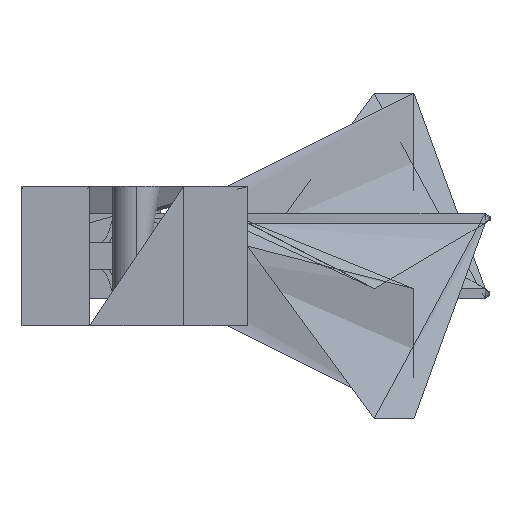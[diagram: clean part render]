
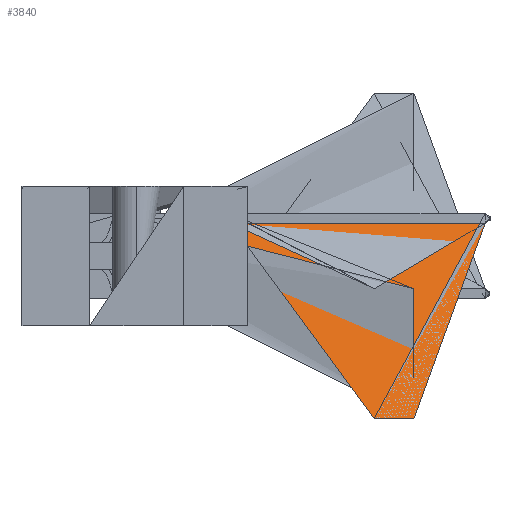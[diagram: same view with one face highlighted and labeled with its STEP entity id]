
A CAD part, left-side view. The second image highlights one B-rep face of the part: STEP entity #3840.
In plain terms, the highlighted face is planar.
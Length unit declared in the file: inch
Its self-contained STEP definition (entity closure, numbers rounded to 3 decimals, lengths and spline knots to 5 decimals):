
#121 = EDGE_CURVE ( 'NONE', #7818, #8210, #23582, .T. ) ;
#2265 = DIRECTION ( 'NONE',  ( -1., 0., 0. ) ) ;
#3840 = ADVANCED_FACE ( 'NONE', ( #11960 ), #12370, .T. ) ;
#4671 = LINE ( 'NONE', #13243, #16494 ) ;
#4996 = CARTESIAN_POINT ( 'NONE',  ( 1.101, 0.558, -0.222 ) ) ;
#5915 = DIRECTION ( 'NONE',  ( 0., 1., 0. ) ) ;
#7014 = VERTEX_POINT ( 'NONE', #4996 ) ;
#7818 = VERTEX_POINT ( 'NONE', #8188 ) ;
#8078 = ORIENTED_EDGE ( 'NONE', *, *, #12349, .F. ) ;
#8188 = CARTESIAN_POINT ( 'NONE',  ( 1.29021, 0.0125, -0.0125 ) ) ;
#8210 = VERTEX_POINT ( 'NONE', #12499 ) ;
#8916 = CARTESIAN_POINT ( 'NONE',  ( 0.61321, 0.0375, -0.0125 ) ) ;
#9231 = EDGE_CURVE ( 'NONE', #7014, #15350, #23465, .T. ) ;
#10148 = VECTOR ( 'NONE', #23608, 39.37008 ) ;
#10782 = VERTEX_POINT ( 'NONE', #14503 ) ;
#11137 = DIRECTION ( 'NONE',  ( -1., 0., 0. ) ) ;
#11462 = ORIENTED_EDGE ( 'NONE', *, *, #22046, .T. ) ;
#11960 = FACE_OUTER_BOUND ( 'NONE', #22001, .T. ) ;
#12349 = EDGE_CURVE ( 'NONE', #10782, #27650, #4671, .T. ) ;
#12370 = PLANE ( 'NONE',  #15108 ) ;
#12499 = CARTESIAN_POINT ( 'NONE',  ( 0.61321, 0.0125, -0.0125 ) ) ;
#12515 = LINE ( 'NONE', #24726, #14184 ) ;
#12797 = ORIENTED_EDGE ( 'NONE', *, *, #121, .T. ) ;
#13243 = CARTESIAN_POINT ( 'NONE',  ( 0.61321, 0.0375, -0.0125 ) ) ;
#14184 = VECTOR ( 'NONE', #5915, 39.37008 ) ;
#14503 = CARTESIAN_POINT ( 'NONE',  ( 1.29021, 0.0375, -0.0125 ) ) ;
#15027 = VECTOR ( 'NONE', #2265, 39.37008 ) ;
#15108 = AXIS2_PLACEMENT_3D ( 'NONE', #16434, #22901, #23168 ) ;
#15350 = VERTEX_POINT ( 'NONE', #15425 ) ;
#15425 = CARTESIAN_POINT ( 'NONE',  ( 0.995, 0.558, -0.222 ) ) ;
#16434 = CARTESIAN_POINT ( 'NONE',  ( 0.61321, -0.71223, -0.0125 ) ) ;
#16494 = VECTOR ( 'NONE', #11137, 39.37008 ) ;
#17673 = ORIENTED_EDGE ( 'NONE', *, *, #9231, .T. ) ;
#22001 = EDGE_LOOP ( 'NONE', ( #8078, #17673, #12797, #11462 ) ) ;
#22046 = EDGE_CURVE ( 'NONE', #8210, #27650, #12515, .T. ) ;
#22901 = DIRECTION ( 'NONE',  ( 0., 0., -1. ) ) ;
#23168 = DIRECTION ( 'NONE',  ( -1., 0., 0. ) ) ;
#23465 = LINE ( 'NONE', #25713, #10148 ) ;
#23582 = LINE ( 'NONE', #25269, #15027 ) ;
#23608 = DIRECTION ( 'NONE',  ( -1., 0., 0. ) ) ;
#24726 = CARTESIAN_POINT ( 'NONE',  ( 0.61321, -0.71223, -0.0125 ) ) ;
#25269 = CARTESIAN_POINT ( 'NONE',  ( 0.61321, 0.0125, -0.0125 ) ) ;
#25713 = CARTESIAN_POINT ( 'NONE',  ( 0.342, 0.558, -0.222 ) ) ;
#27650 = VERTEX_POINT ( 'NONE', #8916 ) ;
